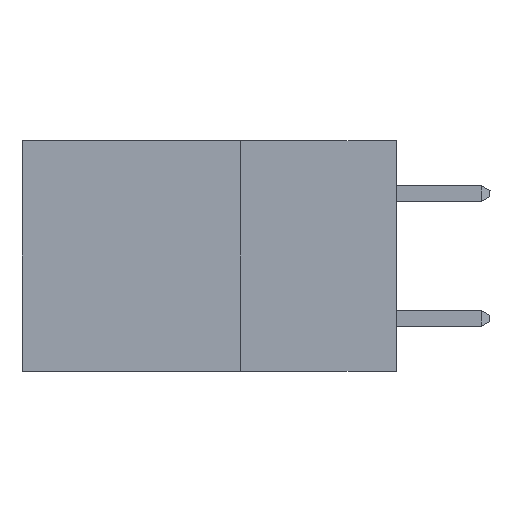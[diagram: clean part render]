
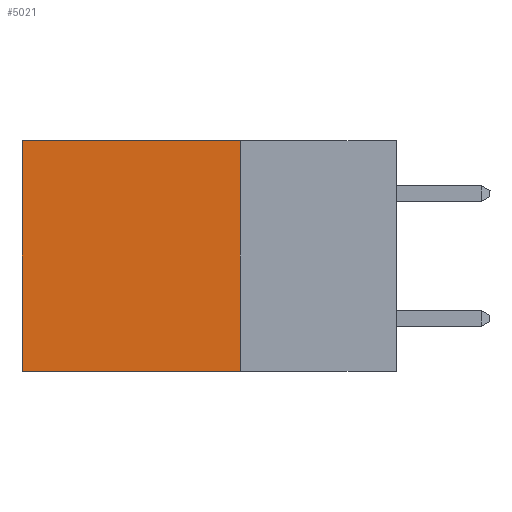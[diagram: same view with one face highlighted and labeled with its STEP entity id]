
A CAD part, left-side view. The second image highlights one B-rep face of the part: STEP entity #5021.
In plain terms, the highlighted planar face has unit normal (-1, 0, 0).
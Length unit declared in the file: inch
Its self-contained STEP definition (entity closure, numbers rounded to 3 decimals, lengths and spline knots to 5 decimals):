
#360 = CARTESIAN_POINT ( 'NONE',  ( 0.298, 0.6, 0. ) ) ;
#438 = CARTESIAN_POINT ( 'NONE',  ( 0.298, 0.25, 0. ) ) ;
#514 = LINE ( 'NONE', #2092, #7300 ) ;
#895 = EDGE_CURVE ( 'NONE', #7418, #6565, #10890, .T. ) ;
#1188 = VECTOR ( 'NONE', #6414, 39.37008 ) ;
#1828 = CARTESIAN_POINT ( 'NONE',  ( 0.298, 0.6, -0.37 ) ) ;
#2092 = CARTESIAN_POINT ( 'NONE',  ( 0.298, 0.25, 0. ) ) ;
#2215 = VECTOR ( 'NONE', #7222, 39.37008 ) ;
#2299 = DIRECTION ( 'NONE',  ( 1., 0., 0. ) ) ;
#2604 = CARTESIAN_POINT ( 'NONE',  ( 0.298, 0.25, 0. ) ) ;
#2867 = VERTEX_POINT ( 'NONE', #11427 ) ;
#3634 = AXIS2_PLACEMENT_3D ( 'NONE', #438, #2299, #8908 ) ;
#4618 = ORIENTED_EDGE ( 'NONE', *, *, #6112, .T. ) ;
#4679 = LINE ( 'NONE', #2604, #2215 ) ;
#4863 = ORIENTED_EDGE ( 'NONE', *, *, #6470, .F. ) ;
#5021 = ADVANCED_FACE ( 'NONE', ( #9322 ), #7805, .F. ) ;
#5988 = LINE ( 'NONE', #8155, #8150 ) ;
#6112 = EDGE_CURVE ( 'NONE', #2867, #7418, #514, .T. ) ;
#6414 = DIRECTION ( 'NONE',  ( 0., 0., -1. ) ) ;
#6470 = EDGE_CURVE ( 'NONE', #10463, #6565, #5988, .T. ) ;
#6565 = VERTEX_POINT ( 'NONE', #1828 ) ;
#6646 = DIRECTION ( 'NONE',  ( 0., 1., 0. ) ) ;
#6730 = EDGE_LOOP ( 'NONE', ( #6758, #4863, #7247, #4618 ) ) ;
#6758 = ORIENTED_EDGE ( 'NONE', *, *, #895, .T. ) ;
#6897 = CARTESIAN_POINT ( 'NONE',  ( 0.298, 0.6, 0. ) ) ;
#7222 = DIRECTION ( 'NONE',  ( 0., 0., -1. ) ) ;
#7247 = ORIENTED_EDGE ( 'NONE', *, *, #7697, .F. ) ;
#7300 = VECTOR ( 'NONE', #6646, 39.37008 ) ;
#7418 = VERTEX_POINT ( 'NONE', #360 ) ;
#7697 = EDGE_CURVE ( 'NONE', #2867, #10463, #4679, .T. ) ;
#7805 = PLANE ( 'NONE',  #3634 ) ;
#8150 = VECTOR ( 'NONE', #9074, 39.37008 ) ;
#8155 = CARTESIAN_POINT ( 'NONE',  ( 0.298, 0.25, -0.37 ) ) ;
#8908 = DIRECTION ( 'NONE',  ( 0., 0., -1. ) ) ;
#9074 = DIRECTION ( 'NONE',  ( 0., 1., 0. ) ) ;
#9322 = FACE_OUTER_BOUND ( 'NONE', #6730, .T. ) ;
#9512 = CARTESIAN_POINT ( 'NONE',  ( 0.298, 0.25, -0.37 ) ) ;
#10463 = VERTEX_POINT ( 'NONE', #9512 ) ;
#10890 = LINE ( 'NONE', #6897, #1188 ) ;
#11427 = CARTESIAN_POINT ( 'NONE',  ( 0.298, 0.25, 0. ) ) ;
